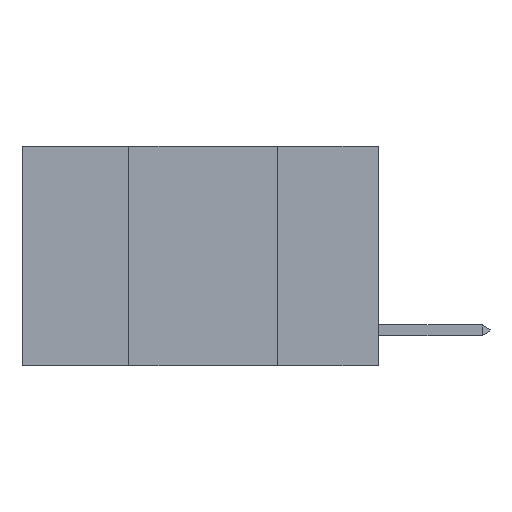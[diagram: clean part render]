
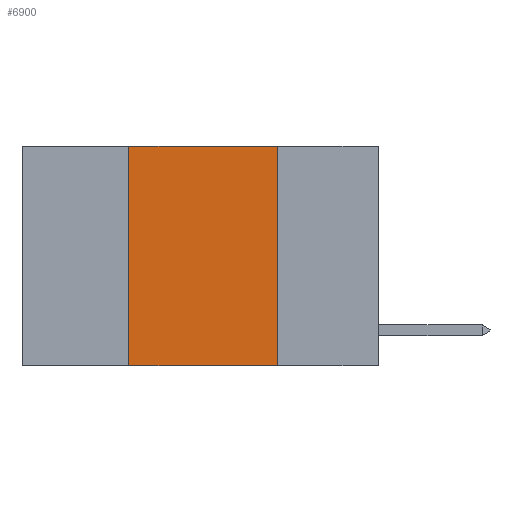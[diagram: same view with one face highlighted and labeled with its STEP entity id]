
A CAD part, left-side view. The second image highlights one B-rep face of the part: STEP entity #6900.
In plain terms, the highlighted planar face has unit normal (-1, 0, 0).
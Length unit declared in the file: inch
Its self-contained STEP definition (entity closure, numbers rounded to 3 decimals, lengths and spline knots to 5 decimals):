
#362 = CARTESIAN_POINT ( 'NONE',  ( 0., 0.17, 0. ) ) ;
#370 = EDGE_LOOP ( 'NONE', ( #6776, #6499, #14967, #1583 ) ) ;
#381 = CARTESIAN_POINT ( 'NONE',  ( 0., 0.6, 0. ) ) ;
#675 = EDGE_CURVE ( 'NONE', #10651, #1109, #1238, .T. ) ;
#1109 = VERTEX_POINT ( 'NONE', #13552 ) ;
#1238 = LINE ( 'NONE', #17763, #2333 ) ;
#1583 = ORIENTED_EDGE ( 'NONE', *, *, #7256, .T. ) ;
#1730 = VECTOR ( 'NONE', #11496, 39.37008 ) ;
#1761 = PLANE ( 'NONE',  #13027 ) ;
#1841 = VECTOR ( 'NONE', #5900, 39.37008 ) ;
#1930 = EDGE_CURVE ( 'NONE', #13921, #10651, #15197, .T. ) ;
#2333 = VECTOR ( 'NONE', #16534, 39.37008 ) ;
#3623 = LINE ( 'NONE', #6207, #3854 ) ;
#3854 = VECTOR ( 'NONE', #16048, 39.37008 ) ;
#4534 = LINE ( 'NONE', #362, #1730 ) ;
#5900 = DIRECTION ( 'NONE',  ( 0., 0., 1. ) ) ;
#6207 = CARTESIAN_POINT ( 'NONE',  ( 0., 0.6, -0.37 ) ) ;
#6499 = ORIENTED_EDGE ( 'NONE', *, *, #675, .F. ) ;
#6776 = ORIENTED_EDGE ( 'NONE', *, *, #16703, .F. ) ;
#6900 = ADVANCED_FACE ( 'NONE', ( #16807 ), #1761, .F. ) ;
#7256 = EDGE_CURVE ( 'NONE', #13921, #12229, #3623, .T. ) ;
#7482 = CARTESIAN_POINT ( 'NONE',  ( 0., 0.42, 0. ) ) ;
#10275 = DIRECTION ( 'NONE',  ( 0., 0., -1. ) ) ;
#10651 = VERTEX_POINT ( 'NONE', #16232 ) ;
#11496 = DIRECTION ( 'NONE',  ( 0., 0., -1. ) ) ;
#12229 = VERTEX_POINT ( 'NONE', #16851 ) ;
#13027 = AXIS2_PLACEMENT_3D ( 'NONE', #381, #14543, #10275 ) ;
#13552 = CARTESIAN_POINT ( 'NONE',  ( 0., 0.17, 0. ) ) ;
#13921 = VERTEX_POINT ( 'NONE', #14471 ) ;
#14471 = CARTESIAN_POINT ( 'NONE',  ( 0., 0.42, -0.37 ) ) ;
#14543 = DIRECTION ( 'NONE',  ( 1., 0., 0. ) ) ;
#14967 = ORIENTED_EDGE ( 'NONE', *, *, #1930, .F. ) ;
#15197 = LINE ( 'NONE', #7482, #1841 ) ;
#16048 = DIRECTION ( 'NONE',  ( 0., -1., 0. ) ) ;
#16232 = CARTESIAN_POINT ( 'NONE',  ( 0., 0.42, 0. ) ) ;
#16534 = DIRECTION ( 'NONE',  ( 0., -1., 0. ) ) ;
#16703 = EDGE_CURVE ( 'NONE', #1109, #12229, #4534, .T. ) ;
#16807 = FACE_OUTER_BOUND ( 'NONE', #370, .T. ) ;
#16851 = CARTESIAN_POINT ( 'NONE',  ( 0., 0.17, -0.37 ) ) ;
#17763 = CARTESIAN_POINT ( 'NONE',  ( 0., 0.6, 0. ) ) ;
